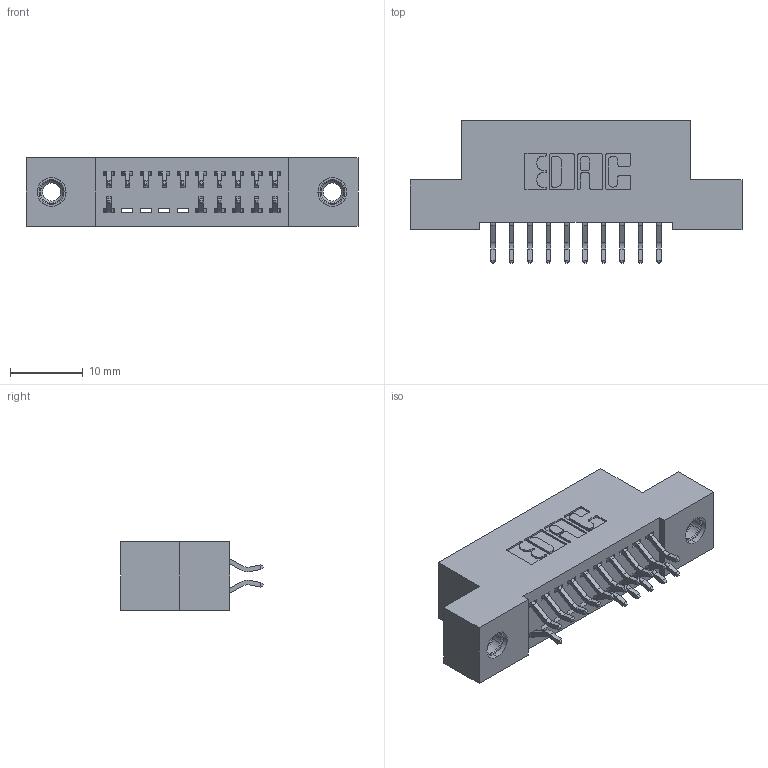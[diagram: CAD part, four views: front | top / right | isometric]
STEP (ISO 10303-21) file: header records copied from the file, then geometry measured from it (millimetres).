
FILE_DESCRIPTION (( 'STEP AP203' ), '1' );
FILE_NAME ('392-020-556-207.STEP', '2018-08-15T07:07:30', ( '' ), ( '' ), 'SwSTEP 2.0', 'SolidWorks 2016', '' );
FILE_SCHEMA (( 'CONFIG_CONTROL_DESIGN' ));
Length unit declared in the file: inch
Products named in the file (4): 342 Part_TI; 345-292-001_556 Tail; 345-250-001_345-250-005-103; 392-020-556-207
Assembly tree (19 placements, depth 2):
  392-020-556-207
    342 Part_TI
    345-292-001_556 Tail  x16
    345-250-001_345-250-005-103  x2
Bounding box: 45.72 x 19.58 x 9.4 mm (x, y, z)
Volume: 3907.4 mm3; surface area: 5383.1 mm2
Topology: 19 solids, 19 shells, 1122 faces, 3287 edges, 2162 vertices
Faces by surface type: plane 762, cylinder 344, cone 12, torus 4
Entity records: 11718 total; most frequent: CARTESIAN_POINT 1993, ORIENTED_EDGE 1914, DIRECTION 1775, EDGE_CURVE 957, VECTOR 801, LINE 801, VERTEX_POINT 632, AXIS2_PLACEMENT_3D 487
